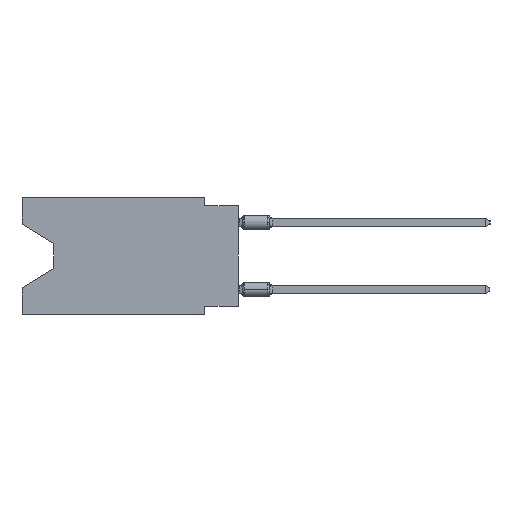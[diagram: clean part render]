
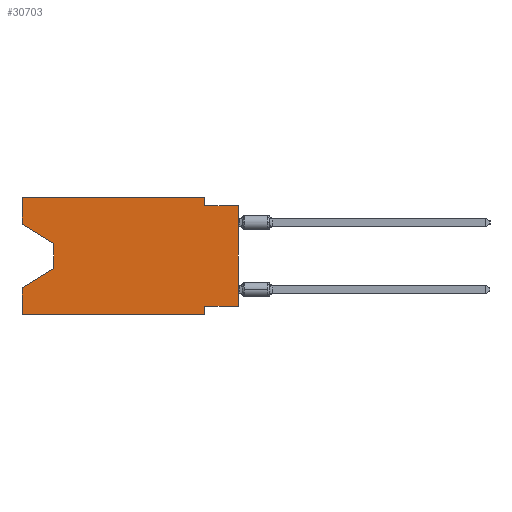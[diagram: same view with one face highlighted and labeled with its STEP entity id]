
A CAD part, left-side view. The second image highlights one B-rep face of the part: STEP entity #30703.
In plain terms, the highlighted planar face has unit normal (-1, 0, 0).
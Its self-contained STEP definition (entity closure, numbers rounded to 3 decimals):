
#229 = EDGE_CURVE ( 'NONE', #27311, #5564, #23720, .T. ) ;
#301 = ORIENTED_EDGE ( 'NONE', *, *, #7781, .T. ) ;
#331 = ORIENTED_EDGE ( 'NONE', *, *, #1143, .F. ) ;
#801 = VECTOR ( 'NONE', #12033, 1000. ) ;
#979 = ORIENTED_EDGE ( 'NONE', *, *, #27302, .F. ) ;
#1143 = EDGE_CURVE ( 'NONE', #21673, #38876, #16463, .T. ) ;
#1466 = CARTESIAN_POINT ( 'NONE',  ( 0., 13.97, -3.505 ) ) ;
#1744 = ORIENTED_EDGE ( 'NONE', *, *, #35530, .F. ) ;
#1799 = CARTESIAN_POINT ( 'NONE',  ( 0., 13.97, -5.385 ) ) ;
#2651 = ORIENTED_EDGE ( 'NONE', *, *, #36749, .T. ) ;
#2846 = VERTEX_POINT ( 'NONE', #4058 ) ;
#4058 = CARTESIAN_POINT ( 'NONE',  ( 0., 16.383, 0. ) ) ;
#4160 = CARTESIAN_POINT ( 'NONE',  ( 0., 2.54, 0. ) ) ;
#4975 = CARTESIAN_POINT ( 'NONE',  ( 0., 16.383, -2.038 ) ) ;
#5210 = ORIENTED_EDGE ( 'NONE', *, *, #229, .T. ) ;
#5564 = VERTEX_POINT ( 'NONE', #8695 ) ;
#5722 = AXIS2_PLACEMENT_3D ( 'NONE', #21582, #6226, #22177 ) ;
#5942 = CARTESIAN_POINT ( 'NONE',  ( 0., 13.97, -5.385 ) ) ;
#5992 = VERTEX_POINT ( 'NONE', #18060 ) ;
#6226 = DIRECTION ( 'NONE',  ( 1., 0., 0. ) ) ;
#6295 = EDGE_CURVE ( 'NONE', #28078, #40195, #14950, .T. ) ;
#6554 = VECTOR ( 'NONE', #35172, 1000. ) ;
#6913 = VECTOR ( 'NONE', #29441, 1000. ) ;
#7569 = LINE ( 'NONE', #29271, #31331 ) ;
#7732 = LINE ( 'NONE', #29860, #35016 ) ;
#7781 = EDGE_CURVE ( 'NONE', #28078, #5992, #14554, .T. ) ;
#8038 = EDGE_CURVE ( 'NONE', #22864, #40195, #20426, .T. ) ;
#8695 = CARTESIAN_POINT ( 'NONE',  ( 0., 0., -0.635 ) ) ;
#10006 = CARTESIAN_POINT ( 'NONE',  ( 0., 16.383, -8.89 ) ) ;
#10031 = VECTOR ( 'NONE', #10311, 1000. ) ;
#10311 = DIRECTION ( 'NONE',  ( 0., 0., -1. ) ) ;
#11046 = DIRECTION ( 'NONE',  ( 0., -0.855, -0.519 ) ) ;
#11388 = DIRECTION ( 'NONE',  ( 0., 0., -1. ) ) ;
#12033 = DIRECTION ( 'NONE',  ( 0., 0., 1. ) ) ;
#14266 = CARTESIAN_POINT ( 'NONE',  ( 0., 0., -8.255 ) ) ;
#14422 = EDGE_CURVE ( 'NONE', #38876, #5564, #7732, .T. ) ;
#14554 = LINE ( 'NONE', #27030, #38952 ) ;
#14781 = ORIENTED_EDGE ( 'NONE', *, *, #14422, .F. ) ;
#14950 = LINE ( 'NONE', #27636, #32966 ) ;
#15274 = VECTOR ( 'NONE', #20359, 1000. ) ;
#15820 = ORIENTED_EDGE ( 'NONE', *, *, #6295, .F. ) ;
#16463 = LINE ( 'NONE', #34703, #10031 ) ;
#16883 = CARTESIAN_POINT ( 'NONE',  ( 0., 2.54, -8.255 ) ) ;
#18060 = CARTESIAN_POINT ( 'NONE',  ( 0., 2.54, -8.89 ) ) ;
#18977 = EDGE_CURVE ( 'NONE', #2846, #21673, #35938, .T. ) ;
#19476 = EDGE_LOOP ( 'NONE', ( #2651, #28940, #40419, #15820, #301, #979, #1744, #5210, #14781, #331, #38709, #23044 ) ) ;
#20359 = DIRECTION ( 'NONE',  ( 0., -1., 0. ) ) ;
#20426 = LINE ( 'NONE', #1799, #6913 ) ;
#21582 = CARTESIAN_POINT ( 'NONE',  ( 0., 16.383, 0. ) ) ;
#21673 = VERTEX_POINT ( 'NONE', #4160 ) ;
#22177 = DIRECTION ( 'NONE',  ( 0., 0., -1. ) ) ;
#22668 = CARTESIAN_POINT ( 'NONE',  ( 0., 13.97, -3.505 ) ) ;
#22864 = VERTEX_POINT ( 'NONE', #5942 ) ;
#23044 = ORIENTED_EDGE ( 'NONE', *, *, #40039, .F. ) ;
#23455 = DIRECTION ( 'NONE',  ( 0., 0., 1. ) ) ;
#23494 = DIRECTION ( 'NONE',  ( 0., -1., 0. ) ) ;
#23666 = CARTESIAN_POINT ( 'NONE',  ( 0., 16.383, 0. ) ) ;
#23720 = LINE ( 'NONE', #30883, #801 ) ;
#23843 = CARTESIAN_POINT ( 'NONE',  ( 0., 16.383, 0. ) ) ;
#24143 = DIRECTION ( 'NONE',  ( 0., -1., 0. ) ) ;
#24868 = CARTESIAN_POINT ( 'NONE',  ( 0., 16.383, -6.852 ) ) ;
#25344 = LINE ( 'NONE', #22668, #6554 ) ;
#25403 = VERTEX_POINT ( 'NONE', #16883 ) ;
#25447 = FACE_OUTER_BOUND ( 'NONE', #19476, .T. ) ;
#27030 = CARTESIAN_POINT ( 'NONE',  ( 0., 16.383, -8.89 ) ) ;
#27276 = VECTOR ( 'NONE', #23455, 1000. ) ;
#27302 = EDGE_CURVE ( 'NONE', #25403, #5992, #28796, .T. ) ;
#27311 = VERTEX_POINT ( 'NONE', #14266 ) ;
#27428 = DIRECTION ( 'NONE',  ( 0., 0., 1. ) ) ;
#27636 = CARTESIAN_POINT ( 'NONE',  ( 0., 16.383, 0. ) ) ;
#27818 = DIRECTION ( 'NONE',  ( 0., 1., 0. ) ) ;
#28078 = VERTEX_POINT ( 'NONE', #10006 ) ;
#28325 = VECTOR ( 'NONE', #27818, 1000. ) ;
#28796 = LINE ( 'NONE', #28995, #29453 ) ;
#28940 = ORIENTED_EDGE ( 'NONE', *, *, #38327, .T. ) ;
#28995 = CARTESIAN_POINT ( 'NONE',  ( 0., 2.54, -8.89 ) ) ;
#29271 = CARTESIAN_POINT ( 'NONE',  ( 0., 16.383, -2.038 ) ) ;
#29441 = DIRECTION ( 'NONE',  ( 0., 0.855, -0.519 ) ) ;
#29453 = VECTOR ( 'NONE', #11388, 1000. ) ;
#29860 = CARTESIAN_POINT ( 'NONE',  ( 0., 0., -0.635 ) ) ;
#30696 = CARTESIAN_POINT ( 'NONE',  ( 0., 0., -8.255 ) ) ;
#30703 = ADVANCED_FACE ( 'NONE', ( #25447 ), #37956, .F. ) ;
#30883 = CARTESIAN_POINT ( 'NONE',  ( 0., 0., 0. ) ) ;
#31331 = VECTOR ( 'NONE', #11046, 1000. ) ;
#32118 = VERTEX_POINT ( 'NONE', #4975 ) ;
#32966 = VECTOR ( 'NONE', #27428, 1000. ) ;
#33729 = VERTEX_POINT ( 'NONE', #1466 ) ;
#34703 = CARTESIAN_POINT ( 'NONE',  ( 0., 2.54, 0. ) ) ;
#35016 = VECTOR ( 'NONE', #23494, 1000. ) ;
#35172 = DIRECTION ( 'NONE',  ( 0., 0., -1. ) ) ;
#35530 = EDGE_CURVE ( 'NONE', #27311, #25403, #39712, .T. ) ;
#35938 = LINE ( 'NONE', #23843, #15274 ) ;
#35956 = CARTESIAN_POINT ( 'NONE',  ( 0., 2.54, -0.635 ) ) ;
#36749 = EDGE_CURVE ( 'NONE', #32118, #33729, #7569, .T. ) ;
#37956 = PLANE ( 'NONE',  #5722 ) ;
#38327 = EDGE_CURVE ( 'NONE', #33729, #22864, #25344, .T. ) ;
#38709 = ORIENTED_EDGE ( 'NONE', *, *, #18977, .F. ) ;
#38817 = LINE ( 'NONE', #23666, #27276 ) ;
#38876 = VERTEX_POINT ( 'NONE', #35956 ) ;
#38952 = VECTOR ( 'NONE', #24143, 1000. ) ;
#39712 = LINE ( 'NONE', #30696, #28325 ) ;
#40039 = EDGE_CURVE ( 'NONE', #32118, #2846, #38817, .T. ) ;
#40195 = VERTEX_POINT ( 'NONE', #24868 ) ;
#40419 = ORIENTED_EDGE ( 'NONE', *, *, #8038, .T. ) ;
